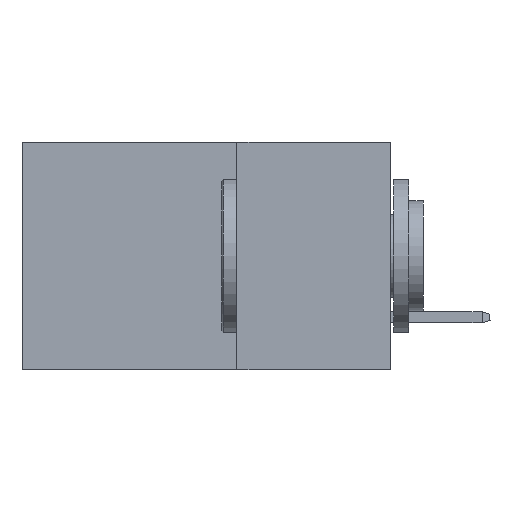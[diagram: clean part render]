
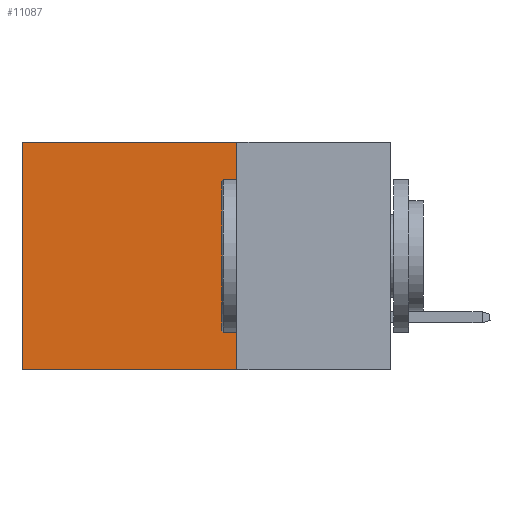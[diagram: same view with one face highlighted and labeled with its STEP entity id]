
A CAD part, left-side view. The second image highlights one B-rep face of the part: STEP entity #11087.
In plain terms, the highlighted planar face has unit normal (-1, 0, 0).
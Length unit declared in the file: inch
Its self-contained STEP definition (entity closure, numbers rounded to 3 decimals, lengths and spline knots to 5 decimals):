
#881 = LINE ( 'NONE', #9738, #30903 ) ;
#918 = CARTESIAN_POINT ( 'NONE',  ( 0.2875, 0.6, -0.37 ) ) ;
#1213 = CARTESIAN_POINT ( 'NONE',  ( 0.2875, 0.25, -0.37 ) ) ;
#1774 = VERTEX_POINT ( 'NONE', #25339 ) ;
#4517 = FACE_OUTER_BOUND ( 'NONE', #27223, .T. ) ;
#4607 = ORIENTED_EDGE ( 'NONE', *, *, #35901, .T. ) ;
#5127 = CARTESIAN_POINT ( 'NONE',  ( 0.2875, 0.6, 0. ) ) ;
#5304 = EDGE_CURVE ( 'NONE', #1774, #21682, #5343, .T. ) ;
#5343 = LINE ( 'NONE', #5127, #8403 ) ;
#6558 = DIRECTION ( 'NONE',  ( 0., 1., 0. ) ) ;
#6800 = ORIENTED_EDGE ( 'NONE', *, *, #22771, .F. ) ;
#7475 = EDGE_CURVE ( 'NONE', #13689, #34997, #881, .T. ) ;
#8403 = VECTOR ( 'NONE', #10491, 39.37008 ) ;
#9596 = CARTESIAN_POINT ( 'NONE',  ( 0.2875, 0.25, 0. ) ) ;
#9738 = CARTESIAN_POINT ( 'NONE',  ( 0.2875, 0.25, 0. ) ) ;
#10491 = DIRECTION ( 'NONE',  ( 0., 0., -1. ) ) ;
#11087 = ADVANCED_FACE ( 'NONE', ( #4517 ), #34700, .F. ) ;
#12663 = DIRECTION ( 'NONE',  ( 0., 0., -1. ) ) ;
#13689 = VERTEX_POINT ( 'NONE', #9596 ) ;
#14977 = CARTESIAN_POINT ( 'NONE',  ( 0.2875, 0.25, 0. ) ) ;
#15195 = DIRECTION ( 'NONE',  ( 0., 1., 0. ) ) ;
#15960 = LINE ( 'NONE', #17599, #21212 ) ;
#17599 = CARTESIAN_POINT ( 'NONE',  ( 0.2875, 0.25, 0. ) ) ;
#18018 = DIRECTION ( 'NONE',  ( 1., 0., 0. ) ) ;
#21212 = VECTOR ( 'NONE', #6558, 39.37008 ) ;
#21682 = VERTEX_POINT ( 'NONE', #918 ) ;
#22771 = EDGE_CURVE ( 'NONE', #34997, #21682, #28966, .T. ) ;
#24568 = CARTESIAN_POINT ( 'NONE',  ( 0.2875, 0.25, -0.37 ) ) ;
#25339 = CARTESIAN_POINT ( 'NONE',  ( 0.2875, 0.6, 0. ) ) ;
#27223 = EDGE_LOOP ( 'NONE', ( #34357, #6800, #30509, #4607 ) ) ;
#28966 = LINE ( 'NONE', #1213, #31576 ) ;
#29001 = DIRECTION ( 'NONE',  ( 0., 0., -1. ) ) ;
#30509 = ORIENTED_EDGE ( 'NONE', *, *, #7475, .F. ) ;
#30903 = VECTOR ( 'NONE', #12663, 39.37008 ) ;
#31576 = VECTOR ( 'NONE', #15195, 39.37008 ) ;
#32414 = AXIS2_PLACEMENT_3D ( 'NONE', #14977, #18018, #29001 ) ;
#34357 = ORIENTED_EDGE ( 'NONE', *, *, #5304, .T. ) ;
#34700 = PLANE ( 'NONE',  #32414 ) ;
#34997 = VERTEX_POINT ( 'NONE', #24568 ) ;
#35901 = EDGE_CURVE ( 'NONE', #13689, #1774, #15960, .T. ) ;
